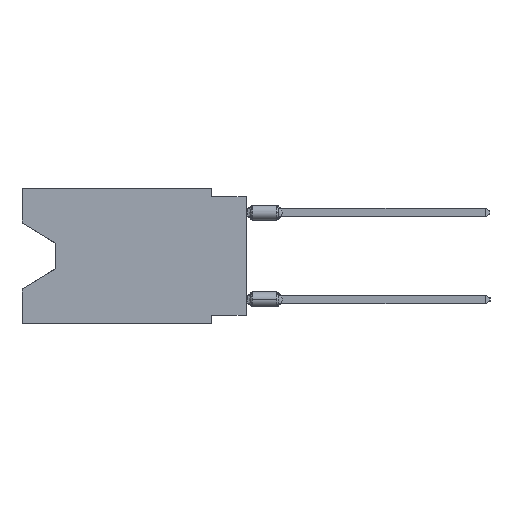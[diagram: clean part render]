
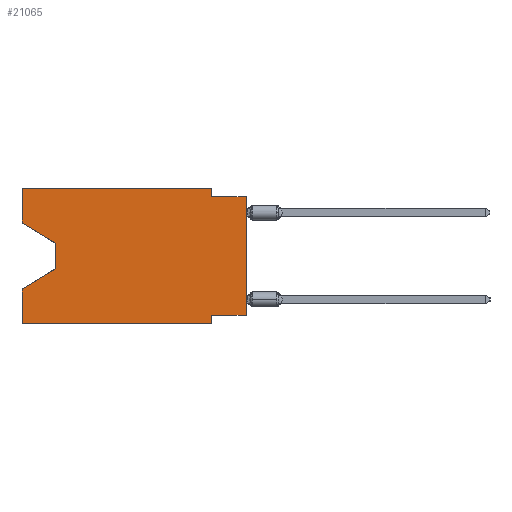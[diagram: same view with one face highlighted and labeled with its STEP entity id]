
A CAD part, left-side view. The second image highlights one B-rep face of the part: STEP entity #21065.
In plain terms, the highlighted planar face has unit normal (-1, 0, 0).
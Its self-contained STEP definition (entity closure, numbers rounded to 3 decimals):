
#183 = EDGE_CURVE ( 'NONE', #49079, #40624, #10601, .T. ) ;
#383 = CARTESIAN_POINT ( 'NONE',  ( 0., 13.97, -5.893 ) ) ;
#630 = EDGE_CURVE ( 'NONE', #41823, #1642, #18449, .T. ) ;
#914 = VECTOR ( 'NONE', #43745, 1000. ) ;
#1278 = VECTOR ( 'NONE', #23292, 1000. ) ;
#1513 = LINE ( 'NONE', #31579, #43032 ) ;
#1642 = VERTEX_POINT ( 'NONE', #23508 ) ;
#2680 = EDGE_CURVE ( 'NONE', #6179, #16550, #39715, .T. ) ;
#2861 = CARTESIAN_POINT ( 'NONE',  ( 0., 16.383, 0. ) ) ;
#3574 = EDGE_CURVE ( 'NONE', #49079, #35163, #30955, .T. ) ;
#3797 = EDGE_CURVE ( 'NONE', #37500, #40624, #37875, .T. ) ;
#4528 = LINE ( 'NONE', #34342, #18454 ) ;
#5790 = AXIS2_PLACEMENT_3D ( 'NONE', #2861, #11236, #6790 ) ;
#5838 = CARTESIAN_POINT ( 'NONE',  ( 0., 2.54, -9.906 ) ) ;
#6179 = VERTEX_POINT ( 'NONE', #16940 ) ;
#6289 = ORIENTED_EDGE ( 'NONE', *, *, #3797, .F. ) ;
#6790 = DIRECTION ( 'NONE',  ( 0., 0., -1. ) ) ;
#6791 = CARTESIAN_POINT ( 'NONE',  ( 0., 2.54, 0. ) ) ;
#7054 = PLANE ( 'NONE',  #5790 ) ;
#8042 = EDGE_CURVE ( 'NONE', #54224, #1642, #12118, .T. ) ;
#8658 = LINE ( 'NONE', #30640, #23242 ) ;
#10286 = LINE ( 'NONE', #5838, #40655 ) ;
#10601 = LINE ( 'NONE', #36499, #42593 ) ;
#11236 = DIRECTION ( 'NONE',  ( 1., 0., 0. ) ) ;
#11557 = CARTESIAN_POINT ( 'NONE',  ( 0., 16.383, 0. ) ) ;
#11894 = VERTEX_POINT ( 'NONE', #27599 ) ;
#12118 = LINE ( 'NONE', #11557, #35061 ) ;
#12789 = CARTESIAN_POINT ( 'NONE',  ( 0., 0., -0.635 ) ) ;
#14338 = DIRECTION ( 'NONE',  ( 0., -0.855, -0.519 ) ) ;
#16550 = VERTEX_POINT ( 'NONE', #52669 ) ;
#16940 = CARTESIAN_POINT ( 'NONE',  ( 0., 16.383, -2.546 ) ) ;
#17863 = CARTESIAN_POINT ( 'NONE',  ( 0., 16.383, 0. ) ) ;
#18148 = ORIENTED_EDGE ( 'NONE', *, *, #183, .T. ) ;
#18449 = LINE ( 'NONE', #383, #45281 ) ;
#18454 = VECTOR ( 'NONE', #30153, 1000. ) ;
#19164 = CARTESIAN_POINT ( 'NONE',  ( 0., 0., -0.635 ) ) ;
#19396 = CARTESIAN_POINT ( 'NONE',  ( 0., 2.54, -9.271 ) ) ;
#19811 = ORIENTED_EDGE ( 'NONE', *, *, #47189, .T. ) ;
#21065 = ADVANCED_FACE ( 'NONE', ( #28481 ), #7054, .F. ) ;
#21403 = DIRECTION ( 'NONE',  ( 0., -1., 0. ) ) ;
#21604 = ORIENTED_EDGE ( 'NONE', *, *, #630, .T. ) ;
#22814 = DIRECTION ( 'NONE',  ( 0., 0., -1. ) ) ;
#23242 = VECTOR ( 'NONE', #29824, 1000. ) ;
#23292 = DIRECTION ( 'NONE',  ( 0., 0., -1. ) ) ;
#23508 = CARTESIAN_POINT ( 'NONE',  ( 0., 16.383, -7.36 ) ) ;
#24660 = ORIENTED_EDGE ( 'NONE', *, *, #2680, .T. ) ;
#25449 = EDGE_CURVE ( 'NONE', #35163, #11894, #10286, .T. ) ;
#26183 = EDGE_CURVE ( 'NONE', #6179, #29661, #4528, .T. ) ;
#26694 = EDGE_LOOP ( 'NONE', ( #24660, #19811, #21604, #34574, #45871, #34200, #50104, #18148, #6289, #46298, #29367, #40259 ) ) ;
#26749 = CARTESIAN_POINT ( 'NONE',  ( 0., 0., -9.271 ) ) ;
#27599 = CARTESIAN_POINT ( 'NONE',  ( 0., 2.54, -9.906 ) ) ;
#28087 = EDGE_CURVE ( 'NONE', #54224, #11894, #1513, .T. ) ;
#28481 = FACE_OUTER_BOUND ( 'NONE', #26694, .T. ) ;
#29367 = ORIENTED_EDGE ( 'NONE', *, *, #43311, .F. ) ;
#29661 = VERTEX_POINT ( 'NONE', #17863 ) ;
#29824 = DIRECTION ( 'NONE',  ( 0., -1., 0. ) ) ;
#30153 = DIRECTION ( 'NONE',  ( 0., 0., 1. ) ) ;
#30640 = CARTESIAN_POINT ( 'NONE',  ( 0., 16.383, 0. ) ) ;
#30955 = LINE ( 'NONE', #26749, #914 ) ;
#31579 = CARTESIAN_POINT ( 'NONE',  ( 0., 16.383, -9.906 ) ) ;
#34200 = ORIENTED_EDGE ( 'NONE', *, *, #25449, .F. ) ;
#34342 = CARTESIAN_POINT ( 'NONE',  ( 0., 16.383, 0. ) ) ;
#34574 = ORIENTED_EDGE ( 'NONE', *, *, #8042, .F. ) ;
#35061 = VECTOR ( 'NONE', #50539, 1000. ) ;
#35163 = VERTEX_POINT ( 'NONE', #19396 ) ;
#35208 = DIRECTION ( 'NONE',  ( 0., -1., 0. ) ) ;
#35240 = CARTESIAN_POINT ( 'NONE',  ( 0., 16.383, -9.906 ) ) ;
#35452 = DIRECTION ( 'NONE',  ( 0., 0.855, -0.519 ) ) ;
#36499 = CARTESIAN_POINT ( 'NONE',  ( 0., 0., 0. ) ) ;
#36736 = VECTOR ( 'NONE', #40366, 1000. ) ;
#37273 = CARTESIAN_POINT ( 'NONE',  ( 0., 13.97, -4.013 ) ) ;
#37500 = VERTEX_POINT ( 'NONE', #45103 ) ;
#37850 = EDGE_CURVE ( 'NONE', #45192, #37500, #40310, .T. ) ;
#37875 = LINE ( 'NONE', #12789, #43612 ) ;
#38394 = CARTESIAN_POINT ( 'NONE',  ( 0., 16.383, -2.546 ) ) ;
#39715 = LINE ( 'NONE', #38394, #52415 ) ;
#40259 = ORIENTED_EDGE ( 'NONE', *, *, #26183, .F. ) ;
#40310 = LINE ( 'NONE', #41118, #1278 ) ;
#40366 = DIRECTION ( 'NONE',  ( 0., 0., -1. ) ) ;
#40624 = VERTEX_POINT ( 'NONE', #19164 ) ;
#40655 = VECTOR ( 'NONE', #22814, 1000. ) ;
#40661 = CARTESIAN_POINT ( 'NONE',  ( 0., 0., -9.271 ) ) ;
#41118 = CARTESIAN_POINT ( 'NONE',  ( 0., 2.54, 0. ) ) ;
#41823 = VERTEX_POINT ( 'NONE', #48202 ) ;
#42593 = VECTOR ( 'NONE', #53751, 1000. ) ;
#43032 = VECTOR ( 'NONE', #35208, 1000. ) ;
#43311 = EDGE_CURVE ( 'NONE', #29661, #45192, #8658, .T. ) ;
#43612 = VECTOR ( 'NONE', #21403, 1000. ) ;
#43745 = DIRECTION ( 'NONE',  ( 0., 1., 0. ) ) ;
#45103 = CARTESIAN_POINT ( 'NONE',  ( 0., 2.54, -0.635 ) ) ;
#45192 = VERTEX_POINT ( 'NONE', #6791 ) ;
#45281 = VECTOR ( 'NONE', #35452, 1000. ) ;
#45871 = ORIENTED_EDGE ( 'NONE', *, *, #28087, .T. ) ;
#46298 = ORIENTED_EDGE ( 'NONE', *, *, #37850, .F. ) ;
#47189 = EDGE_CURVE ( 'NONE', #16550, #41823, #48981, .T. ) ;
#48202 = CARTESIAN_POINT ( 'NONE',  ( 0., 13.97, -5.893 ) ) ;
#48981 = LINE ( 'NONE', #37273, #36736 ) ;
#49079 = VERTEX_POINT ( 'NONE', #40661 ) ;
#50104 = ORIENTED_EDGE ( 'NONE', *, *, #3574, .F. ) ;
#50539 = DIRECTION ( 'NONE',  ( 0., 0., 1. ) ) ;
#52415 = VECTOR ( 'NONE', #14338, 1000. ) ;
#52669 = CARTESIAN_POINT ( 'NONE',  ( 0., 13.97, -4.013 ) ) ;
#53751 = DIRECTION ( 'NONE',  ( 0., 0., 1. ) ) ;
#54224 = VERTEX_POINT ( 'NONE', #35240 ) ;
